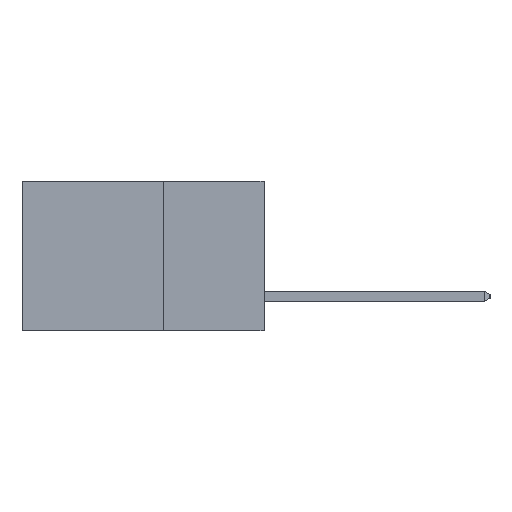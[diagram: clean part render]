
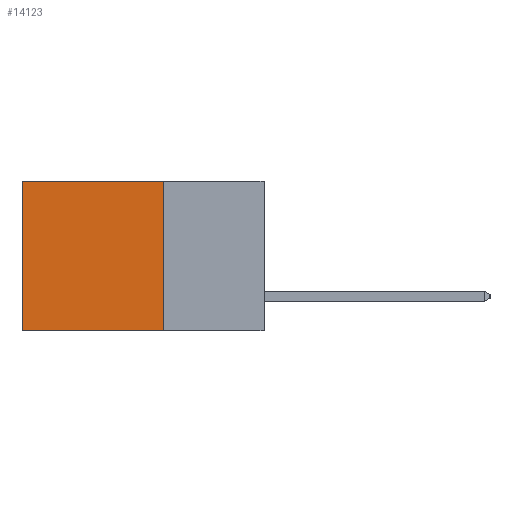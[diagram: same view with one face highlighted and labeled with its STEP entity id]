
A CAD part, left-side view. The second image highlights one B-rep face of the part: STEP entity #14123.
In plain terms, the highlighted planar face has unit normal (-1, 0, 0).
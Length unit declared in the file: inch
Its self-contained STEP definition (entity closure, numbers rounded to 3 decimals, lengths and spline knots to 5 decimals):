
#167 = ORIENTED_EDGE ( 'NONE', *, *, #17037, .T. ) ;
#414 = CARTESIAN_POINT ( 'NONE',  ( 0.2615, 0.25, -0.37 ) ) ;
#608 = VERTEX_POINT ( 'NONE', #3444 ) ;
#1679 = VECTOR ( 'NONE', #3766, 39.37008 ) ;
#2573 = DIRECTION ( 'NONE',  ( 0., 0., -1. ) ) ;
#2591 = DIRECTION ( 'NONE',  ( 1., 0., 0. ) ) ;
#2656 = PLANE ( 'NONE',  #6297 ) ;
#2985 = CARTESIAN_POINT ( 'NONE',  ( 0.2615, 0.25, -0.37 ) ) ;
#3444 = CARTESIAN_POINT ( 'NONE',  ( 0.2615, 0.25, 0. ) ) ;
#3766 = DIRECTION ( 'NONE',  ( 0., 1., 0. ) ) ;
#4042 = CARTESIAN_POINT ( 'NONE',  ( 0.2615, 0.25, -0.37 ) ) ;
#6292 = VERTEX_POINT ( 'NONE', #13708 ) ;
#6297 = AXIS2_PLACEMENT_3D ( 'NONE', #2985, #2591, #2573 ) ;
#6348 = EDGE_CURVE ( 'NONE', #6292, #18274, #18472, .T. ) ;
#6481 = DIRECTION ( 'NONE',  ( 0., 0., -1. ) ) ;
#6535 = CARTESIAN_POINT ( 'NONE',  ( 0.2615, 0.25, -0.37 ) ) ;
#8297 = VERTEX_POINT ( 'NONE', #414 ) ;
#8504 = ORIENTED_EDGE ( 'NONE', *, *, #13740, .F. ) ;
#9230 = DIRECTION ( 'NONE',  ( 0., 1., 0. ) ) ;
#9453 = CARTESIAN_POINT ( 'NONE',  ( 0.2615, 0.25, 0. ) ) ;
#9662 = ORIENTED_EDGE ( 'NONE', *, *, #6348, .T. ) ;
#9774 = VECTOR ( 'NONE', #10266, 39.37008 ) ;
#10266 = DIRECTION ( 'NONE',  ( 0., 0., -1. ) ) ;
#10786 = LINE ( 'NONE', #6535, #18936 ) ;
#11184 = LINE ( 'NONE', #4042, #1679 ) ;
#11272 = FACE_OUTER_BOUND ( 'NONE', #15520, .T. ) ;
#11866 = CARTESIAN_POINT ( 'NONE',  ( 0.2615, 0.6, -0.37 ) ) ;
#13708 = CARTESIAN_POINT ( 'NONE',  ( 0.2615, 0.6, 0. ) ) ;
#13740 = EDGE_CURVE ( 'NONE', #608, #8297, #10786, .T. ) ;
#14094 = ORIENTED_EDGE ( 'NONE', *, *, #15690, .F. ) ;
#14123 = ADVANCED_FACE ( 'NONE', ( #11272 ), #2656, .F. ) ;
#15520 = EDGE_LOOP ( 'NONE', ( #9662, #14094, #8504, #167 ) ) ;
#15690 = EDGE_CURVE ( 'NONE', #8297, #18274, #11184, .T. ) ;
#16758 = LINE ( 'NONE', #9453, #17261 ) ;
#17037 = EDGE_CURVE ( 'NONE', #608, #6292, #16758, .T. ) ;
#17261 = VECTOR ( 'NONE', #9230, 39.37008 ) ;
#17609 = CARTESIAN_POINT ( 'NONE',  ( 0.2615, 0.6, -0.37 ) ) ;
#18274 = VERTEX_POINT ( 'NONE', #17609 ) ;
#18472 = LINE ( 'NONE', #11866, #9774 ) ;
#18936 = VECTOR ( 'NONE', #6481, 39.37008 ) ;
